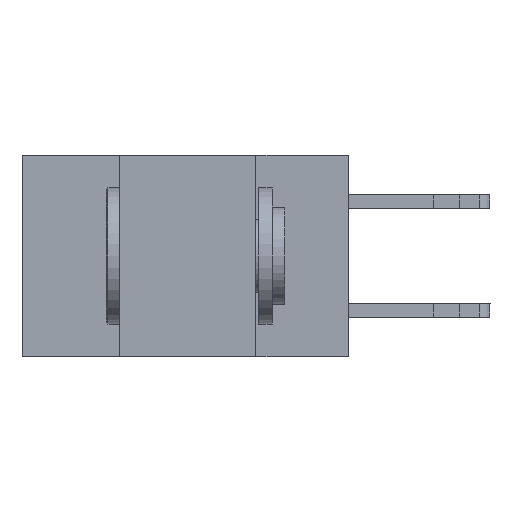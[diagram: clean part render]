
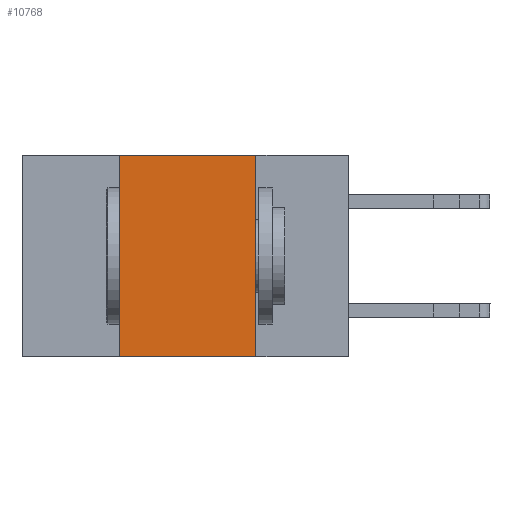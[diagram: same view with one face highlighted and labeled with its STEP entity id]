
A CAD part, left-side view. The second image highlights one B-rep face of the part: STEP entity #10768.
In plain terms, the highlighted planar face has unit normal (-1, 0, 0).
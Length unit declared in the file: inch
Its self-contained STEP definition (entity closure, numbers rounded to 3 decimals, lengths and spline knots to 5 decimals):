
#157 = CARTESIAN_POINT ( 'NONE',  ( 0., 0.17, 0. ) ) ;
#823 = ORIENTED_EDGE ( 'NONE', *, *, #4347, .F. ) ;
#1360 = VECTOR ( 'NONE', #16880, 39.37008 ) ;
#1807 = LINE ( 'NONE', #16765, #1360 ) ;
#2599 = VERTEX_POINT ( 'NONE', #16502 ) ;
#3840 = DIRECTION ( 'NONE',  ( 0., 0., 1. ) ) ;
#4347 = EDGE_CURVE ( 'NONE', #12258, #14046, #13016, .T. ) ;
#5054 = FACE_OUTER_BOUND ( 'NONE', #13512, .T. ) ;
#5196 = DIRECTION ( 'NONE',  ( 0., -1., 0. ) ) ;
#5424 = PLANE ( 'NONE',  #15999 ) ;
#5717 = ORIENTED_EDGE ( 'NONE', *, *, #11972, .F. ) ;
#6103 = VERTEX_POINT ( 'NONE', #15860 ) ;
#6353 = LINE ( 'NONE', #11995, #13585 ) ;
#6492 = LINE ( 'NONE', #17116, #13305 ) ;
#6730 = DIRECTION ( 'NONE',  ( 1., 0., 0. ) ) ;
#6856 = ORIENTED_EDGE ( 'NONE', *, *, #9202, .F. ) ;
#7353 = EDGE_CURVE ( 'NONE', #6103, #14046, #1807, .T. ) ;
#7441 = ORIENTED_EDGE ( 'NONE', *, *, #7353, .T. ) ;
#8948 = VECTOR ( 'NONE', #14555, 39.37008 ) ;
#9202 = EDGE_CURVE ( 'NONE', #6103, #2599, #6353, .T. ) ;
#10768 = ADVANCED_FACE ( 'NONE', ( #5054 ), #5424, .F. ) ;
#11972 = EDGE_CURVE ( 'NONE', #2599, #12258, #6492, .T. ) ;
#11995 = CARTESIAN_POINT ( 'NONE',  ( 0., 0.42, -0.37 ) ) ;
#12258 = VERTEX_POINT ( 'NONE', #157 ) ;
#12301 = CARTESIAN_POINT ( 'NONE',  ( 0., 0.17, -0.37 ) ) ;
#13016 = LINE ( 'NONE', #15164, #8948 ) ;
#13305 = VECTOR ( 'NONE', #5196, 39.37008 ) ;
#13512 = EDGE_LOOP ( 'NONE', ( #823, #5717, #6856, #7441 ) ) ;
#13525 = CARTESIAN_POINT ( 'NONE',  ( 0., 0.6, 0. ) ) ;
#13585 = VECTOR ( 'NONE', #3840, 39.37008 ) ;
#14046 = VERTEX_POINT ( 'NONE', #12301 ) ;
#14555 = DIRECTION ( 'NONE',  ( 0., 0., -1. ) ) ;
#15164 = CARTESIAN_POINT ( 'NONE',  ( 0., 0.17, -0.37 ) ) ;
#15860 = CARTESIAN_POINT ( 'NONE',  ( 0., 0.42, -0.37 ) ) ;
#15999 = AXIS2_PLACEMENT_3D ( 'NONE', #13525, #6730, #16100 ) ;
#16100 = DIRECTION ( 'NONE',  ( 0., 0., -1. ) ) ;
#16502 = CARTESIAN_POINT ( 'NONE',  ( 0., 0.42, 0. ) ) ;
#16765 = CARTESIAN_POINT ( 'NONE',  ( 0., 0.6, -0.37 ) ) ;
#16880 = DIRECTION ( 'NONE',  ( 0., -1., 0. ) ) ;
#17116 = CARTESIAN_POINT ( 'NONE',  ( 0., 0.6, 0. ) ) ;
